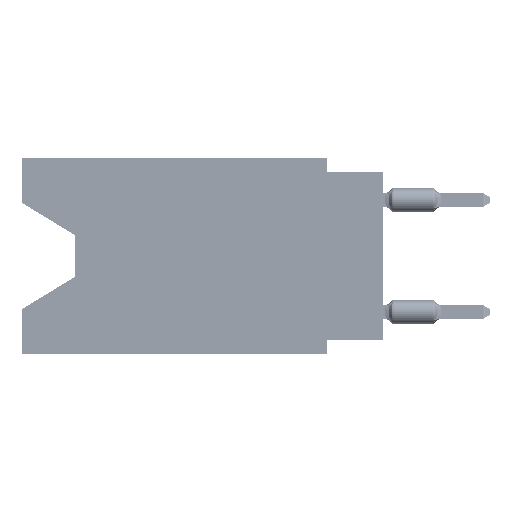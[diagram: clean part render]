
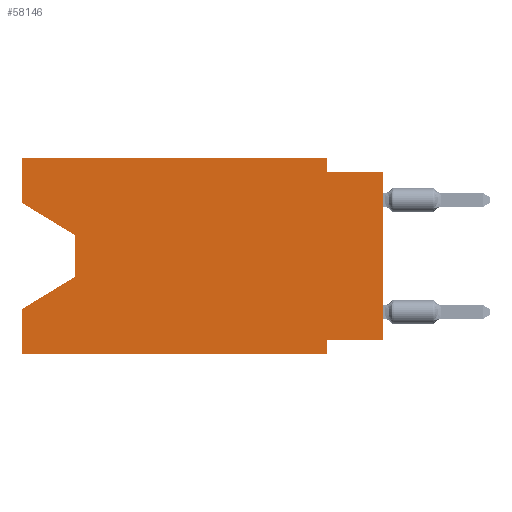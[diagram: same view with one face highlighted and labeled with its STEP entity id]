
A CAD part, left-side view. The second image highlights one B-rep face of the part: STEP entity #58146.
In plain terms, the highlighted planar face has unit normal (-1, 0, 0).
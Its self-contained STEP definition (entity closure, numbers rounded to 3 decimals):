
#182 = LINE ( 'NONE', #14393, #68569 ) ;
#325 = LINE ( 'NONE', #13673, #53874 ) ;
#454 = CARTESIAN_POINT ( 'NONE',  ( 0., 13.97, -5.385 ) ) ;
#659 = ORIENTED_EDGE ( 'NONE', *, *, #63258, .T. ) ;
#741 = EDGE_CURVE ( 'NONE', #50782, #19631, #30228, .T. ) ;
#1010 = DIRECTION ( 'NONE',  ( 0., -0.855, -0.519 ) ) ;
#1014 = FACE_OUTER_BOUND ( 'NONE', #57436, .T. ) ;
#1358 = DIRECTION ( 'NONE',  ( 0., 0., 1. ) ) ;
#3257 = ORIENTED_EDGE ( 'NONE', *, *, #34065, .F. ) ;
#3680 = CARTESIAN_POINT ( 'NONE',  ( 0., 0., -8.255 ) ) ;
#4811 = LINE ( 'NONE', #12799, #84997 ) ;
#6816 = CARTESIAN_POINT ( 'NONE',  ( 0., 16.383, 0. ) ) ;
#6858 = DIRECTION ( 'NONE',  ( 0., 0., -1. ) ) ;
#6890 = DIRECTION ( 'NONE',  ( 0., -1., 0. ) ) ;
#7047 = CARTESIAN_POINT ( 'NONE',  ( 0., 0., -0.635 ) ) ;
#7692 = DIRECTION ( 'NONE',  ( 1., 0., 0. ) ) ;
#7764 = LINE ( 'NONE', #33987, #12289 ) ;
#8033 = VECTOR ( 'NONE', #66164, 1000. ) ;
#8548 = VECTOR ( 'NONE', #44297, 1000. ) ;
#8776 = EDGE_CURVE ( 'NONE', #50782, #79260, #4811, .T. ) ;
#9637 = VERTEX_POINT ( 'NONE', #86579 ) ;
#10591 = EDGE_CURVE ( 'NONE', #59332, #64486, #76946, .T. ) ;
#12289 = VECTOR ( 'NONE', #6890, 1000. ) ;
#12799 = CARTESIAN_POINT ( 'NONE',  ( 0., 0., 0. ) ) ;
#13673 = CARTESIAN_POINT ( 'NONE',  ( 0., 16.383, -8.89 ) ) ;
#14393 = CARTESIAN_POINT ( 'NONE',  ( 0., 2.54, 0. ) ) ;
#15290 = EDGE_CURVE ( 'NONE', #40406, #24686, #182, .T. ) ;
#15669 = CARTESIAN_POINT ( 'NONE',  ( 0., 16.383, -8.89 ) ) ;
#15990 = VECTOR ( 'NONE', #17776, 1000. ) ;
#17670 = ORIENTED_EDGE ( 'NONE', *, *, #18499, .T. ) ;
#17776 = DIRECTION ( 'NONE',  ( 0., 1., 0. ) ) ;
#18235 = VERTEX_POINT ( 'NONE', #23126 ) ;
#18499 = EDGE_CURVE ( 'NONE', #79655, #57170, #29130, .T. ) ;
#18614 = VECTOR ( 'NONE', #1358, 1000. ) ;
#19572 = LINE ( 'NONE', #454, #8033 ) ;
#19631 = VERTEX_POINT ( 'NONE', #73681 ) ;
#19719 = VECTOR ( 'NONE', #39915, 1000. ) ;
#22226 = ORIENTED_EDGE ( 'NONE', *, *, #56649, .F. ) ;
#22657 = LINE ( 'NONE', #39703, #18614 ) ;
#23126 = CARTESIAN_POINT ( 'NONE',  ( 0., 2.54, -8.89 ) ) ;
#24686 = VERTEX_POINT ( 'NONE', #74004 ) ;
#26122 = ORIENTED_EDGE ( 'NONE', *, *, #69239, .T. ) ;
#26158 = VECTOR ( 'NONE', #1010, 1000. ) ;
#28098 = PLANE ( 'NONE',  #82411 ) ;
#28544 = DIRECTION ( 'NONE',  ( 0., 0., -1. ) ) ;
#29130 = LINE ( 'NONE', #56209, #70551 ) ;
#30100 = ORIENTED_EDGE ( 'NONE', *, *, #15290, .F. ) ;
#30228 = LINE ( 'NONE', #65261, #15990 ) ;
#33987 = CARTESIAN_POINT ( 'NONE',  ( 0., 16.383, 0. ) ) ;
#34065 = EDGE_CURVE ( 'NONE', #78383, #9637, #22657, .T. ) ;
#34498 = DIRECTION ( 'NONE',  ( 0., 0., -1. ) ) ;
#34769 = CARTESIAN_POINT ( 'NONE',  ( 0., 16.383, -2.038 ) ) ;
#38773 = DIRECTION ( 'NONE',  ( 0., 0., 1. ) ) ;
#39078 = ORIENTED_EDGE ( 'NONE', *, *, #8776, .T. ) ;
#39703 = CARTESIAN_POINT ( 'NONE',  ( 0., 16.383, 0. ) ) ;
#39915 = DIRECTION ( 'NONE',  ( 0., -1., 0. ) ) ;
#40254 = EDGE_CURVE ( 'NONE', #9637, #40406, #7764, .T. ) ;
#40406 = VERTEX_POINT ( 'NONE', #64104 ) ;
#40549 = CARTESIAN_POINT ( 'NONE',  ( 0., 13.97, -3.505 ) ) ;
#42692 = VECTOR ( 'NONE', #38773, 1000. ) ;
#43857 = CARTESIAN_POINT ( 'NONE',  ( 0., 2.54, -8.89 ) ) ;
#44297 = DIRECTION ( 'NONE',  ( 0., 0., -1. ) ) ;
#45427 = CARTESIAN_POINT ( 'NONE',  ( 0., 16.383, 0. ) ) ;
#47414 = DIRECTION ( 'NONE',  ( 0., -1., 0. ) ) ;
#49392 = LINE ( 'NONE', #34769, #26158 ) ;
#49908 = CARTESIAN_POINT ( 'NONE',  ( 0., 16.383, -2.038 ) ) ;
#50782 = VERTEX_POINT ( 'NONE', #3680 ) ;
#52293 = ORIENTED_EDGE ( 'NONE', *, *, #55060, .F. ) ;
#53332 = LINE ( 'NONE', #7047, #19719 ) ;
#53874 = VECTOR ( 'NONE', #47414, 1000. ) ;
#55060 = EDGE_CURVE ( 'NONE', #24686, #79260, #53332, .T. ) ;
#56209 = CARTESIAN_POINT ( 'NONE',  ( 0., 13.97, -3.505 ) ) ;
#56649 = EDGE_CURVE ( 'NONE', #19631, #18235, #57168, .T. ) ;
#57168 = LINE ( 'NONE', #43857, #8548 ) ;
#57170 = VERTEX_POINT ( 'NONE', #82225 ) ;
#57436 = EDGE_LOOP ( 'NONE', ( #659, #17670, #26122, #81514, #81201, #22226, #65778, #39078, #52293, #30100, #65918, #3257 ) ) ;
#58146 = ADVANCED_FACE ( 'NONE', ( #1014 ), #28098, .F. ) ;
#59332 = VERTEX_POINT ( 'NONE', #15669 ) ;
#63258 = EDGE_CURVE ( 'NONE', #78383, #79655, #49392, .T. ) ;
#64104 = CARTESIAN_POINT ( 'NONE',  ( 0., 2.54, 0. ) ) ;
#64486 = VERTEX_POINT ( 'NONE', #70236 ) ;
#65261 = CARTESIAN_POINT ( 'NONE',  ( 0., 0., -8.255 ) ) ;
#65778 = ORIENTED_EDGE ( 'NONE', *, *, #741, .F. ) ;
#65918 = ORIENTED_EDGE ( 'NONE', *, *, #40254, .F. ) ;
#66164 = DIRECTION ( 'NONE',  ( 0., 0.855, -0.519 ) ) ;
#66930 = DIRECTION ( 'NONE',  ( 0., 0., 1. ) ) ;
#68569 = VECTOR ( 'NONE', #6858, 1000. ) ;
#69239 = EDGE_CURVE ( 'NONE', #57170, #64486, #19572, .T. ) ;
#70236 = CARTESIAN_POINT ( 'NONE',  ( 0., 16.383, -6.852 ) ) ;
#70551 = VECTOR ( 'NONE', #34498, 1000. ) ;
#73681 = CARTESIAN_POINT ( 'NONE',  ( 0., 2.54, -8.255 ) ) ;
#74004 = CARTESIAN_POINT ( 'NONE',  ( 0., 2.54, -0.635 ) ) ;
#76946 = LINE ( 'NONE', #45427, #42692 ) ;
#78383 = VERTEX_POINT ( 'NONE', #49908 ) ;
#79260 = VERTEX_POINT ( 'NONE', #81011 ) ;
#79655 = VERTEX_POINT ( 'NONE', #40549 ) ;
#81011 = CARTESIAN_POINT ( 'NONE',  ( 0., 0., -0.635 ) ) ;
#81201 = ORIENTED_EDGE ( 'NONE', *, *, #81805, .T. ) ;
#81514 = ORIENTED_EDGE ( 'NONE', *, *, #10591, .F. ) ;
#81805 = EDGE_CURVE ( 'NONE', #59332, #18235, #325, .T. ) ;
#82225 = CARTESIAN_POINT ( 'NONE',  ( 0., 13.97, -5.385 ) ) ;
#82411 = AXIS2_PLACEMENT_3D ( 'NONE', #6816, #7692, #28544 ) ;
#84997 = VECTOR ( 'NONE', #66930, 1000. ) ;
#86579 = CARTESIAN_POINT ( 'NONE',  ( 0., 16.383, 0. ) ) ;
